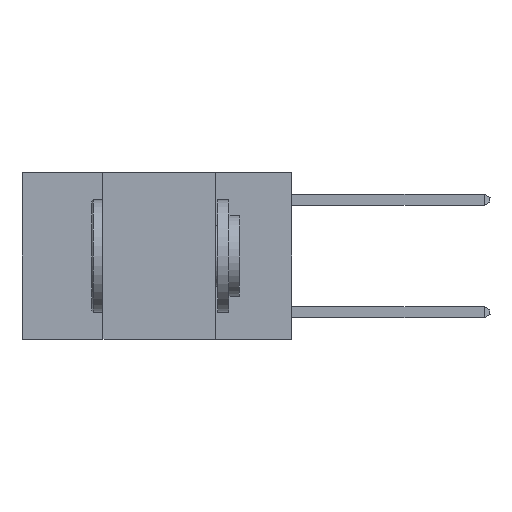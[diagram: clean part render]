
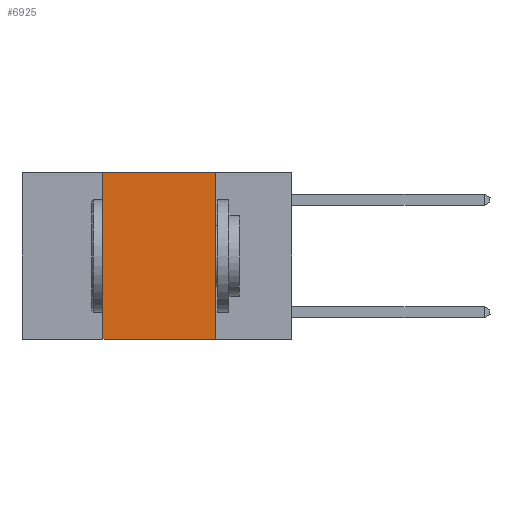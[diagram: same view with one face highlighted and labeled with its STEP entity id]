
A CAD part, left-side view. The second image highlights one B-rep face of the part: STEP entity #6925.
In plain terms, the highlighted planar face has unit normal (-1, 0, 0).
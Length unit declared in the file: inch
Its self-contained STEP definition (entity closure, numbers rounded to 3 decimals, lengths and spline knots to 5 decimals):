
#123 = VECTOR ( 'NONE', #15423, 39.37008 ) ;
#847 = EDGE_CURVE ( 'NONE', #18009, #18172, #17042, .T. ) ;
#1837 = DIRECTION ( 'NONE',  ( 0., -1., 0. ) ) ;
#2016 = ORIENTED_EDGE ( 'NONE', *, *, #847, .F. ) ;
#2550 = VECTOR ( 'NONE', #21464, 39.37008 ) ;
#2703 = VERTEX_POINT ( 'NONE', #19373 ) ;
#2834 = LINE ( 'NONE', #19830, #9265 ) ;
#3436 = DIRECTION ( 'NONE',  ( 0., 0., -1. ) ) ;
#4551 = LINE ( 'NONE', #19569, #2550 ) ;
#6916 = ORIENTED_EDGE ( 'NONE', *, *, #11672, .F. ) ;
#6925 = ADVANCED_FACE ( 'NONE', ( #12128 ), #10003, .F. ) ;
#7272 = CARTESIAN_POINT ( 'NONE',  ( 0., 0.17, 0. ) ) ;
#8606 = CARTESIAN_POINT ( 'NONE',  ( 0., 0.6, 0. ) ) ;
#9265 = VECTOR ( 'NONE', #13187, 39.37008 ) ;
#10003 = PLANE ( 'NONE',  #17158 ) ;
#11466 = ORIENTED_EDGE ( 'NONE', *, *, #13907, .T. ) ;
#11672 = EDGE_CURVE ( 'NONE', #2703, #18009, #2834, .T. ) ;
#11678 = CARTESIAN_POINT ( 'NONE',  ( 0., 0.6, 0. ) ) ;
#12128 = FACE_OUTER_BOUND ( 'NONE', #21815, .T. ) ;
#13187 = DIRECTION ( 'NONE',  ( 0., 0., 1. ) ) ;
#13475 = ORIENTED_EDGE ( 'NONE', *, *, #14684, .F. ) ;
#13907 = EDGE_CURVE ( 'NONE', #2703, #15767, #4551, .T. ) ;
#14684 = EDGE_CURVE ( 'NONE', #18172, #15767, #17288, .T. ) ;
#15192 = VECTOR ( 'NONE', #1837, 39.37008 ) ;
#15423 = DIRECTION ( 'NONE',  ( 0., 0., -1. ) ) ;
#15767 = VERTEX_POINT ( 'NONE', #16840 ) ;
#16801 = CARTESIAN_POINT ( 'NONE',  ( 0., 0.17, 0. ) ) ;
#16840 = CARTESIAN_POINT ( 'NONE',  ( 0., 0.17, -0.37 ) ) ;
#17042 = LINE ( 'NONE', #8606, #15192 ) ;
#17158 = AXIS2_PLACEMENT_3D ( 'NONE', #11678, #18879, #3436 ) ;
#17288 = LINE ( 'NONE', #7272, #123 ) ;
#18009 = VERTEX_POINT ( 'NONE', #20978 ) ;
#18172 = VERTEX_POINT ( 'NONE', #16801 ) ;
#18879 = DIRECTION ( 'NONE',  ( 1., 0., 0. ) ) ;
#19373 = CARTESIAN_POINT ( 'NONE',  ( 0., 0.42, -0.37 ) ) ;
#19569 = CARTESIAN_POINT ( 'NONE',  ( 0., 0.6, -0.37 ) ) ;
#19830 = CARTESIAN_POINT ( 'NONE',  ( 0., 0.42, 0. ) ) ;
#20978 = CARTESIAN_POINT ( 'NONE',  ( 0., 0.42, 0. ) ) ;
#21464 = DIRECTION ( 'NONE',  ( 0., -1., 0. ) ) ;
#21815 = EDGE_LOOP ( 'NONE', ( #13475, #2016, #6916, #11466 ) ) ;
